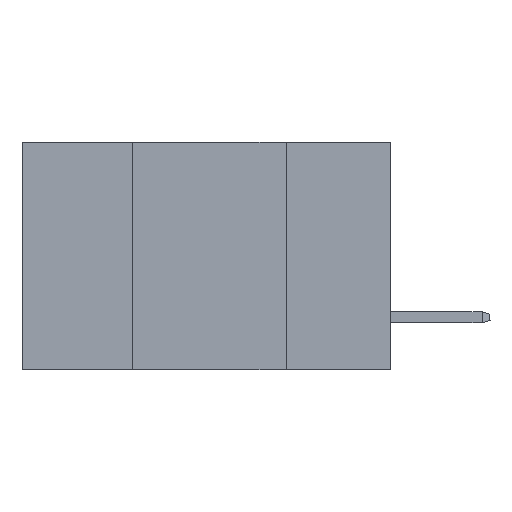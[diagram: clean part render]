
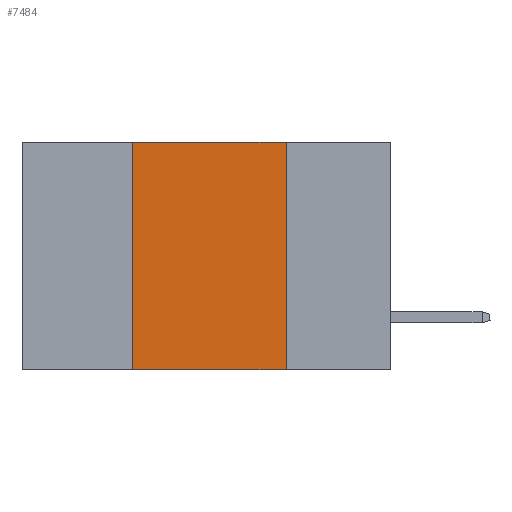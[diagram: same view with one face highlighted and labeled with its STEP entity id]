
A CAD part, left-side view. The second image highlights one B-rep face of the part: STEP entity #7484.
In plain terms, the highlighted planar face has unit normal (-1, 0, 0).
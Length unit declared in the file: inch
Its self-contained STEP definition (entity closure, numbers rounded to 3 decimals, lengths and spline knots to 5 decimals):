
#328 = LINE ( 'NONE', #22334, #16576 ) ;
#892 = EDGE_CURVE ( 'NONE', #20134, #19156, #21185, .T. ) ;
#1411 = DIRECTION ( 'NONE',  ( 0., -1., 0. ) ) ;
#2134 = CARTESIAN_POINT ( 'NONE',  ( 0., 0.17, 0. ) ) ;
#2309 = CARTESIAN_POINT ( 'NONE',  ( 0., 0.17, 0. ) ) ;
#2481 = ORIENTED_EDGE ( 'NONE', *, *, #20913, .F. ) ;
#3364 = ORIENTED_EDGE ( 'NONE', *, *, #892, .F. ) ;
#6454 = EDGE_LOOP ( 'NONE', ( #15540, #3364, #2481, #18215 ) ) ;
#7484 = ADVANCED_FACE ( 'NONE', ( #15309 ), #20647, .F. ) ;
#7711 = EDGE_CURVE ( 'NONE', #8165, #7921, #17492, .T. ) ;
#7921 = VERTEX_POINT ( 'NONE', #19556 ) ;
#8165 = VERTEX_POINT ( 'NONE', #17287 ) ;
#8645 = DIRECTION ( 'NONE',  ( 0., 0., 1. ) ) ;
#9964 = CARTESIAN_POINT ( 'NONE',  ( 0., 0.6, 0. ) ) ;
#10680 = DIRECTION ( 'NONE',  ( 0., 0., -1. ) ) ;
#11432 = DIRECTION ( 'NONE',  ( 0., -1., 0. ) ) ;
#11992 = DIRECTION ( 'NONE',  ( 1., 0., 0. ) ) ;
#12785 = LINE ( 'NONE', #2309, #17964 ) ;
#13317 = CARTESIAN_POINT ( 'NONE',  ( 0., 0.42, 0. ) ) ;
#13852 = CARTESIAN_POINT ( 'NONE',  ( 0., 0.6, -0.37 ) ) ;
#13940 = EDGE_CURVE ( 'NONE', #19156, #7921, #12785, .T. ) ;
#14166 = DIRECTION ( 'NONE',  ( 0., 0., -1. ) ) ;
#15309 = FACE_OUTER_BOUND ( 'NONE', #6454, .T. ) ;
#15540 = ORIENTED_EDGE ( 'NONE', *, *, #13940, .F. ) ;
#16576 = VECTOR ( 'NONE', #8645, 39.37008 ) ;
#17287 = CARTESIAN_POINT ( 'NONE',  ( 0., 0.42, -0.37 ) ) ;
#17492 = LINE ( 'NONE', #13852, #18049 ) ;
#17920 = VECTOR ( 'NONE', #11432, 39.37008 ) ;
#17964 = VECTOR ( 'NONE', #10680, 39.37008 ) ;
#18049 = VECTOR ( 'NONE', #1411, 39.37008 ) ;
#18215 = ORIENTED_EDGE ( 'NONE', *, *, #7711, .T. ) ;
#19156 = VERTEX_POINT ( 'NONE', #2134 ) ;
#19556 = CARTESIAN_POINT ( 'NONE',  ( 0., 0.17, -0.37 ) ) ;
#20134 = VERTEX_POINT ( 'NONE', #13317 ) ;
#20204 = AXIS2_PLACEMENT_3D ( 'NONE', #9964, #11992, #14166 ) ;
#20300 = CARTESIAN_POINT ( 'NONE',  ( 0., 0.6, 0. ) ) ;
#20647 = PLANE ( 'NONE',  #20204 ) ;
#20913 = EDGE_CURVE ( 'NONE', #8165, #20134, #328, .T. ) ;
#21185 = LINE ( 'NONE', #20300, #17920 ) ;
#22334 = CARTESIAN_POINT ( 'NONE',  ( 0., 0.42, 0. ) ) ;
